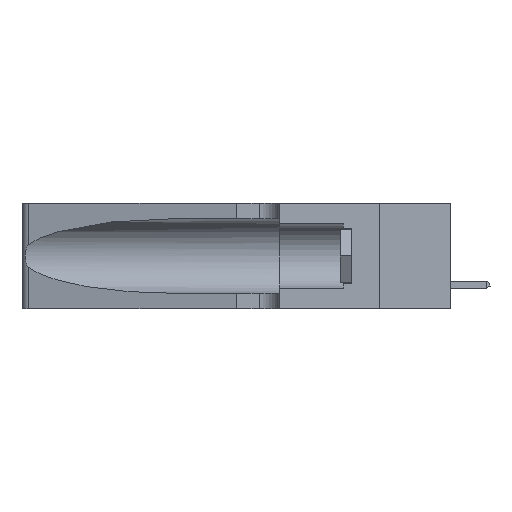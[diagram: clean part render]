
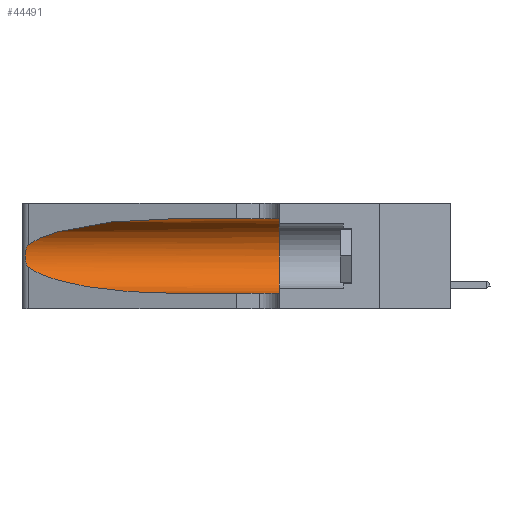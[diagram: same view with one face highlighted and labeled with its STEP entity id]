
A CAD part, left-side view. The second image highlights one B-rep face of the part: STEP entity #44491.
In plain terms, the highlighted cylindrical face has radius 3.308 mm (diameter 6.617 mm), a partial arc.
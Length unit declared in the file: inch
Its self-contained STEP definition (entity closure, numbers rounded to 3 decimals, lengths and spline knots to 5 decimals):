
#1070 = VERTEX_POINT ( 'NONE', #13613 ) ;
#1872 = CARTESIAN_POINT ( 'NONE',  ( 0.1305, 1.61858, 0.185 ) ) ;
#3834 = CARTESIAN_POINT ( 'NONE',  ( 0.2373, 1.15595, 0.28018 ) ) ;
#5032 = CARTESIAN_POINT ( 'NONE',  ( 0.26018, 1.23835, 0.19895 ) ) ;
#5993 = VECTOR ( 'NONE', #37719, 39.37008 ) ;
#6355 = FACE_OUTER_BOUND ( 'NONE', #12464, .T. ) ;
#8380 = DIRECTION ( 'NONE',  ( 0., -1., 0. ) ) ;
#8460 = CARTESIAN_POINT ( 'NONE',  ( 0.1305, 0.35, 0.31525 ) ) ;
#8536 = CARTESIAN_POINT ( 'NONE',  ( 0.26075, 1.23896, 0.178 ) ) ;
#12019 = CARTESIAN_POINT ( 'NONE',  ( 0.25856, 1.23593, 0.16098 ) ) ;
#12025 = DIRECTION ( 'NONE',  ( 0., 0., -1. ) ) ;
#12165 = CARTESIAN_POINT ( 'NONE',  ( 0.25639, 1.23186, 0.15144 ) ) ;
#12464 = EDGE_LOOP ( 'NONE', ( #24383, #41082, #13804, #44167, #38126, #36043 ) ) ;
#13538 = VERTEX_POINT ( 'NONE', #23520 ) ;
#13613 = CARTESIAN_POINT ( 'NONE',  ( 0.1305, 0.72297, 0.31525 ) ) ;
#13804 = ORIENTED_EDGE ( 'NONE', *, *, #34033, .T. ) ;
#16503 = VERTEX_POINT ( 'NONE', #8460 ) ;
#17176 = CYLINDRICAL_SURFACE ( 'NONE', #28713, 0.13025 ) ;
#17237 = CARTESIAN_POINT ( 'NONE',  ( 0.25487, 1.22718, 0.14631 ) ) ;
#17955 = LINE ( 'NONE', #30744, #5993 ) ;
#18435 = CARTESIAN_POINT ( 'NONE',  ( 0.1305, 0.35, 0.05475 ) ) ;
#19093 = CARTESIAN_POINT ( 'NONE',  ( 0.26017, 1.23833, 0.17102 ) ) ;
#20039 = AXIS2_PLACEMENT_3D ( 'NONE', #31899, #24586, #27947 ) ;
#20610 = CARTESIAN_POINT ( 'NONE',  ( 0.25487, 1.22718, 0.22369 ) ) ;
#23122 = CARTESIAN_POINT ( 'NONE',  ( 0.2373, 1.15595, 0.08982 ) ) ;
#23520 = CARTESIAN_POINT ( 'NONE',  ( 0.1305, 0.72297, 0.05475 ) ) ;
#24383 = ORIENTED_EDGE ( 'NONE', *, *, #26208, .T. ) ;
#24415 = EDGE_CURVE ( 'NONE', #13538, #24846, #17955, .T. ) ;
#24586 = DIRECTION ( 'NONE',  ( 0., 1., 0. ) ) ;
#24668 = VECTOR ( 'NONE', #32060, 39.37008 ) ;
#24846 = VERTEX_POINT ( 'NONE', #18435 ) ;
#25207 = CARTESIAN_POINT ( 'NONE',  ( 0.1305, 1.61858, 0.31525 ) ) ;
#25267 = EDGE_CURVE ( 'NONE', #16503, #24846, #31158, .T. ) ;
#25628 = CARTESIAN_POINT ( 'NONE',  ( 0.25789, 1.23486, 0.15765 ) ) ;
#25746 = LINE ( 'NONE', #25207, #24668 ) ;
#25784 = CARTESIAN_POINT ( 'NONE',  ( 0.25854, 1.2359, 0.20912 ) ) ;
#26208 = EDGE_CURVE ( 'NONE', #1070, #42611, #31677, .T. ) ;
#27756 = B_SPLINE_CURVE_WITH_KNOTS ( 'NONE', 3,
 ( #43066, #29427, #35956, #39609, #25784, #5032, #29279, #8536, #19093, #12019, #25628, #12165, #36261, #39755 ),
 .UNSPECIFIED., .F., .F.,
 ( 4, 2, 2, 2, 2, 2, 4 ),
 ( 0., 0.00027, 0.00053, 0.00107, 0.0016, 0.00187, 0.00214 ),
 .UNSPECIFIED. ) ;
#27947 = DIRECTION ( 'NONE',  ( 0., 0., 1. ) ) ;
#28713 = AXIS2_PLACEMENT_3D ( 'NONE', #1872, #8380, #12025 ) ;
#29279 = CARTESIAN_POINT ( 'NONE',  ( 0.26075, 1.23896, 0.19203 ) ) ;
#29427 = CARTESIAN_POINT ( 'NONE',  ( 0.25555, 1.22994, 0.2215 ) ) ;
#30721 = CARTESIAN_POINT ( 'NONE',  ( 0.1305, 0.72297, 0.05475 ) ) ;
#30744 = CARTESIAN_POINT ( 'NONE',  ( 0.1305, 1.61858, 0.05475 ) ) ;
#30969 = CARTESIAN_POINT ( 'NONE',  ( 0.18966, 0.96281, 0.31525 ) ) ;
#31158 = CIRCLE ( 'NONE', #20039, 0.13025 ) ;
#31172 = EDGE_CURVE ( 'NONE', #1070, #16503, #25746, .T. ) ;
#31347 = CARTESIAN_POINT ( 'NONE',  ( 0.25487, 1.22718, 0.22369 ) ) ;
#31677 =( BOUNDED_CURVE ( )  B_SPLINE_CURVE ( 3, ( #41423, #30969, #3834, #20610 ),
 .UNSPECIFIED., .F., .T. ) 
 B_SPLINE_CURVE_WITH_KNOTS ( ( 4, 4 ),
 ( 1.5708, 2.84003 ),
 .UNSPECIFIED. ) 
 CURVE ( )  GEOMETRIC_REPRESENTATION_ITEM ( )  RATIONAL_B_SPLINE_CURVE ( ( 1., 0.87, 0.87, 1. ) ) 
 REPRESENTATION_ITEM ( '' )  );
#31899 = CARTESIAN_POINT ( 'NONE',  ( 0.1305, 0.35, 0.185 ) ) ;
#32060 = DIRECTION ( 'NONE',  ( 0., -1., 0. ) ) ;
#34033 = EDGE_CURVE ( 'NONE', #42585, #13538, #43044, .T. ) ;
#34354 = CARTESIAN_POINT ( 'NONE',  ( 0.18966, 0.96281, 0.05475 ) ) ;
#35956 = CARTESIAN_POINT ( 'NONE',  ( 0.25639, 1.23184, 0.21858 ) ) ;
#36043 = ORIENTED_EDGE ( 'NONE', *, *, #31172, .F. ) ;
#36261 = CARTESIAN_POINT ( 'NONE',  ( 0.25555, 1.22993, 0.14849 ) ) ;
#37719 = DIRECTION ( 'NONE',  ( 0., -1., 0. ) ) ;
#38126 = ORIENTED_EDGE ( 'NONE', *, *, #25267, .F. ) ;
#39577 = EDGE_CURVE ( 'NONE', #42611, #42585, #27756, .T. ) ;
#39609 = CARTESIAN_POINT ( 'NONE',  ( 0.25787, 1.23484, 0.2124 ) ) ;
#39755 = CARTESIAN_POINT ( 'NONE',  ( 0.25487, 1.22718, 0.14631 ) ) ;
#40863 = CARTESIAN_POINT ( 'NONE',  ( 0.25487, 1.22718, 0.14631 ) ) ;
#41082 = ORIENTED_EDGE ( 'NONE', *, *, #39577, .T. ) ;
#41423 = CARTESIAN_POINT ( 'NONE',  ( 0.1305, 0.72297, 0.31525 ) ) ;
#42585 = VERTEX_POINT ( 'NONE', #17237 ) ;
#42611 = VERTEX_POINT ( 'NONE', #31347 ) ;
#43044 =( BOUNDED_CURVE ( )  B_SPLINE_CURVE ( 3, ( #40863, #23122, #34354, #30721 ),
 .UNSPECIFIED., .F., .T. ) 
 B_SPLINE_CURVE_WITH_KNOTS ( ( 4, 4 ),
 ( 3.44316, 4.71239 ),
 .UNSPECIFIED. ) 
 CURVE ( )  GEOMETRIC_REPRESENTATION_ITEM ( )  RATIONAL_B_SPLINE_CURVE ( ( 1., 0.87, 0.87, 1. ) ) 
 REPRESENTATION_ITEM ( '' )  );
#43066 = CARTESIAN_POINT ( 'NONE',  ( 0.25487, 1.22718, 0.22369 ) ) ;
#44167 = ORIENTED_EDGE ( 'NONE', *, *, #24415, .T. ) ;
#44491 = ADVANCED_FACE ( 'NONE', ( #6355 ), #17176, .F. ) ;
